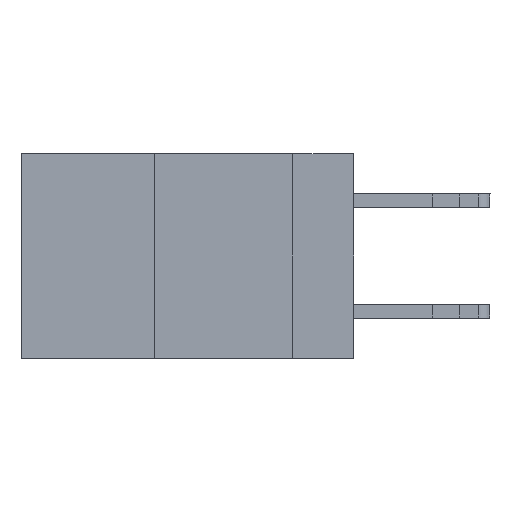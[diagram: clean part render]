
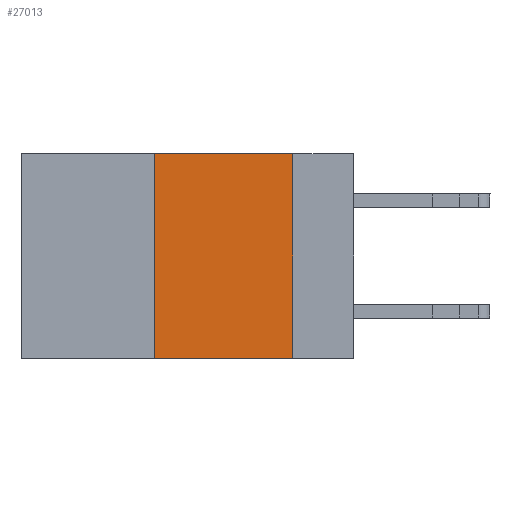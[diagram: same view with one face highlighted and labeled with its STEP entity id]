
A CAD part, left-side view. The second image highlights one B-rep face of the part: STEP entity #27013.
In plain terms, the highlighted planar face has unit normal (-1, 0, 0).
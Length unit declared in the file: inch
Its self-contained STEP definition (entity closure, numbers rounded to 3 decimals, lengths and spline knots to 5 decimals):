
#620 = LINE ( 'NONE', #2289, #9876 ) ;
#974 = LINE ( 'NONE', #15465, #14851 ) ;
#2289 = CARTESIAN_POINT ( 'NONE',  ( 0., 0.6, -0.37 ) ) ;
#2688 = EDGE_CURVE ( 'NONE', #33630, #17466, #620, .T. ) ;
#3664 = DIRECTION ( 'NONE',  ( 0., 0., 1. ) ) ;
#3918 = PLANE ( 'NONE',  #32685 ) ;
#6784 = CARTESIAN_POINT ( 'NONE',  ( 0., 0.11, 0. ) ) ;
#9876 = VECTOR ( 'NONE', #20968, 39.37008 ) ;
#10971 = CARTESIAN_POINT ( 'NONE',  ( 0., 0.6, 0. ) ) ;
#11634 = VECTOR ( 'NONE', #21364, 39.37008 ) ;
#12113 = ORIENTED_EDGE ( 'NONE', *, *, #19136, .F. ) ;
#12160 = LINE ( 'NONE', #10971, #33759 ) ;
#14566 = EDGE_LOOP ( 'NONE', ( #26039, #12113, #35451, #29148 ) ) ;
#14598 = VERTEX_POINT ( 'NONE', #37678 ) ;
#14851 = VECTOR ( 'NONE', #3664, 39.37008 ) ;
#15465 = CARTESIAN_POINT ( 'NONE',  ( 0., 0.36, 0. ) ) ;
#16485 = CARTESIAN_POINT ( 'NONE',  ( 0., 0.11, -0.37 ) ) ;
#17466 = VERTEX_POINT ( 'NONE', #16485 ) ;
#19136 = EDGE_CURVE ( 'NONE', #14598, #23425, #12160, .T. ) ;
#20230 = DIRECTION ( 'NONE',  ( 0., -1., 0. ) ) ;
#20968 = DIRECTION ( 'NONE',  ( 0., -1., 0. ) ) ;
#21337 = EDGE_CURVE ( 'NONE', #33630, #14598, #974, .T. ) ;
#21338 = EDGE_CURVE ( 'NONE', #23425, #17466, #24946, .T. ) ;
#21364 = DIRECTION ( 'NONE',  ( 0., 0., -1. ) ) ;
#23425 = VERTEX_POINT ( 'NONE', #37565 ) ;
#24946 = LINE ( 'NONE', #6784, #11634 ) ;
#26039 = ORIENTED_EDGE ( 'NONE', *, *, #21338, .F. ) ;
#27013 = ADVANCED_FACE ( 'NONE', ( #29757 ), #3918, .F. ) ;
#29148 = ORIENTED_EDGE ( 'NONE', *, *, #2688, .T. ) ;
#29757 = FACE_OUTER_BOUND ( 'NONE', #14566, .T. ) ;
#30436 = DIRECTION ( 'NONE',  ( 0., 0., -1. ) ) ;
#32678 = CARTESIAN_POINT ( 'NONE',  ( 0., 0.36, -0.37 ) ) ;
#32685 = AXIS2_PLACEMENT_3D ( 'NONE', #33377, #35387, #30436 ) ;
#33377 = CARTESIAN_POINT ( 'NONE',  ( 0., 0.6, 0. ) ) ;
#33630 = VERTEX_POINT ( 'NONE', #32678 ) ;
#33759 = VECTOR ( 'NONE', #20230, 39.37008 ) ;
#35387 = DIRECTION ( 'NONE',  ( 1., 0., 0. ) ) ;
#35451 = ORIENTED_EDGE ( 'NONE', *, *, #21337, .F. ) ;
#37565 = CARTESIAN_POINT ( 'NONE',  ( 0., 0.11, 0. ) ) ;
#37678 = CARTESIAN_POINT ( 'NONE',  ( 0., 0.36, 0. ) ) ;
